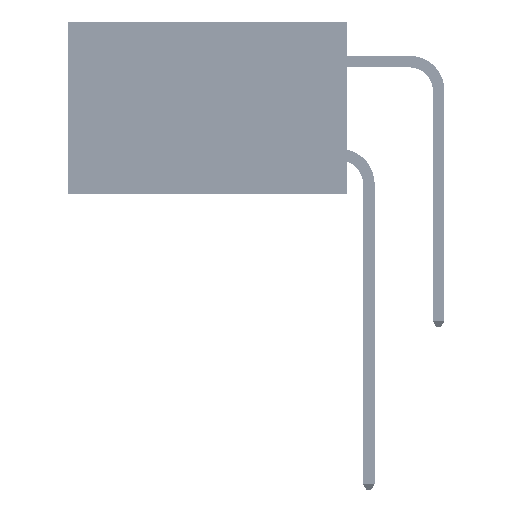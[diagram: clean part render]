
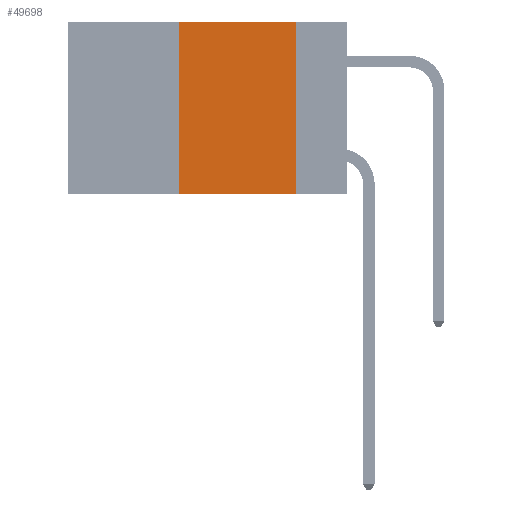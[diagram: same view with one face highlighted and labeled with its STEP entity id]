
A CAD part, left-side view. The second image highlights one B-rep face of the part: STEP entity #49698.
In plain terms, the highlighted planar face has unit normal (-1, 0, 0).
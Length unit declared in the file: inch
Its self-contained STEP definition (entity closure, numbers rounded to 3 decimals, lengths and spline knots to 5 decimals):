
#1463 = CARTESIAN_POINT ( 'NONE',  ( 0., 0.6, 0. ) ) ;
#2968 = VECTOR ( 'NONE', #14203, 39.37008 ) ;
#3230 = AXIS2_PLACEMENT_3D ( 'NONE', #1463, #41056, #37556 ) ;
#6545 = ORIENTED_EDGE ( 'NONE', *, *, #33324, .F. ) ;
#8887 = CARTESIAN_POINT ( 'NONE',  ( 0., 0.6, 0. ) ) ;
#9601 = LINE ( 'NONE', #31657, #42002 ) ;
#10988 = ORIENTED_EDGE ( 'NONE', *, *, #11105, .T. ) ;
#11105 = EDGE_CURVE ( 'NONE', #42408, #46805, #13212, .T. ) ;
#11715 = VERTEX_POINT ( 'NONE', #45732 ) ;
#13212 = LINE ( 'NONE', #37701, #25023 ) ;
#14203 = DIRECTION ( 'NONE',  ( 0., 0., 1. ) ) ;
#18005 = DIRECTION ( 'NONE',  ( 0., -1., 0. ) ) ;
#23772 = EDGE_CURVE ( 'NONE', #49549, #46805, #9601, .T. ) ;
#24314 = CARTESIAN_POINT ( 'NONE',  ( 0., 0.11, 0. ) ) ;
#24472 = FACE_OUTER_BOUND ( 'NONE', #26232, .T. ) ;
#25023 = VECTOR ( 'NONE', #18005, 39.37008 ) ;
#25399 = ORIENTED_EDGE ( 'NONE', *, *, #23772, .F. ) ;
#26232 = EDGE_LOOP ( 'NONE', ( #25399, #45502, #6545, #10988 ) ) ;
#28400 = DIRECTION ( 'NONE',  ( 0., -1., 0. ) ) ;
#30925 = CARTESIAN_POINT ( 'NONE',  ( 0., 0.11, -0.37 ) ) ;
#31657 = CARTESIAN_POINT ( 'NONE',  ( 0., 0.11, 0. ) ) ;
#32421 = VECTOR ( 'NONE', #28400, 39.37008 ) ;
#33324 = EDGE_CURVE ( 'NONE', #42408, #11715, #39803, .T. ) ;
#34222 = CARTESIAN_POINT ( 'NONE',  ( 0., 0.36, 0. ) ) ;
#37481 = CARTESIAN_POINT ( 'NONE',  ( 0., 0.36, -0.37 ) ) ;
#37556 = DIRECTION ( 'NONE',  ( 0., 0., -1. ) ) ;
#37701 = CARTESIAN_POINT ( 'NONE',  ( 0., 0.6, -0.37 ) ) ;
#39496 = DIRECTION ( 'NONE',  ( 0., 0., -1. ) ) ;
#39803 = LINE ( 'NONE', #34222, #2968 ) ;
#41056 = DIRECTION ( 'NONE',  ( 1., 0., 0. ) ) ;
#42002 = VECTOR ( 'NONE', #39496, 39.37008 ) ;
#42408 = VERTEX_POINT ( 'NONE', #37481 ) ;
#43286 = EDGE_CURVE ( 'NONE', #11715, #49549, #50533, .T. ) ;
#45037 = PLANE ( 'NONE',  #3230 ) ;
#45502 = ORIENTED_EDGE ( 'NONE', *, *, #43286, .F. ) ;
#45732 = CARTESIAN_POINT ( 'NONE',  ( 0., 0.36, 0. ) ) ;
#46805 = VERTEX_POINT ( 'NONE', #30925 ) ;
#49549 = VERTEX_POINT ( 'NONE', #24314 ) ;
#49698 = ADVANCED_FACE ( 'NONE', ( #24472 ), #45037, .F. ) ;
#50533 = LINE ( 'NONE', #8887, #32421 ) ;
